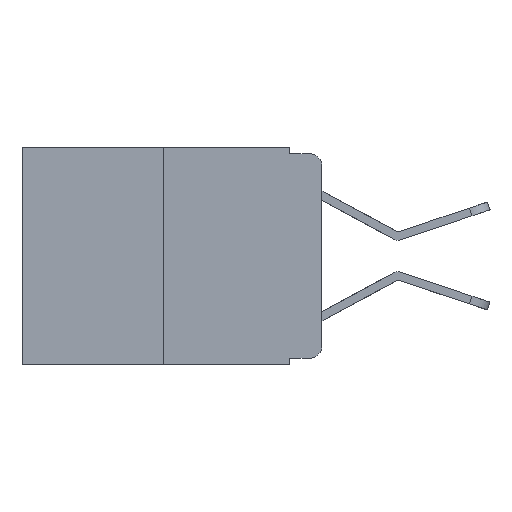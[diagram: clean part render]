
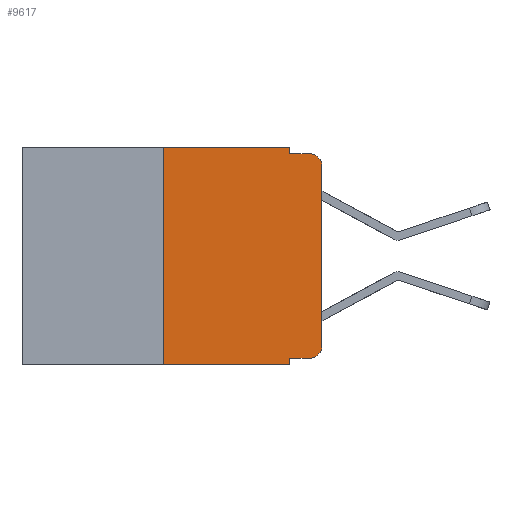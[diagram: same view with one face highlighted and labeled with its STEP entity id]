
A CAD part, left-side view. The second image highlights one B-rep face of the part: STEP entity #9617.
In plain terms, the highlighted planar face has unit normal (-1, 0, 0).
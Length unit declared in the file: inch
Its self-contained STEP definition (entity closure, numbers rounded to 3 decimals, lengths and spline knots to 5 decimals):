
#63 = EDGE_CURVE ( 'NONE', #12526, #5836, #4943, .T. ) ;
#164 = CARTESIAN_POINT ( 'NONE',  ( 0., 0.051, -0.333 ) ) ;
#312 = CIRCLE ( 'NONE', #6295, 0.02 ) ;
#563 = EDGE_CURVE ( 'NONE', #21910, #14165, #8749, .T. ) ;
#1496 = VERTEX_POINT ( 'NONE', #6691 ) ;
#2004 = ORIENTED_EDGE ( 'NONE', *, *, #4461, .T. ) ;
#2182 = VERTEX_POINT ( 'NONE', #14511 ) ;
#2661 = EDGE_CURVE ( 'NONE', #5836, #21910, #312, .T. ) ;
#2753 = DIRECTION ( 'NONE',  ( 1., 0., 0. ) ) ;
#2936 = ORIENTED_EDGE ( 'NONE', *, *, #20538, .F. ) ;
#3021 = CARTESIAN_POINT ( 'NONE',  ( 0., 0.02, -0.01 ) ) ;
#3452 = CARTESIAN_POINT ( 'NONE',  ( 0., 0.473, -0.343 ) ) ;
#3718 = VECTOR ( 'NONE', #7671, 39.37008 ) ;
#3837 = ORIENTED_EDGE ( 'NONE', *, *, #11950, .F. ) ;
#4069 = VECTOR ( 'NONE', #9968, 39.37008 ) ;
#4179 = DIRECTION ( 'NONE',  ( 0., -1., 0. ) ) ;
#4271 = CARTESIAN_POINT ( 'NONE',  ( 0., 0., 0. ) ) ;
#4301 = CARTESIAN_POINT ( 'NONE',  ( 0., 0.051, -0.01 ) ) ;
#4461 = EDGE_CURVE ( 'NONE', #14165, #23490, #7382, .T. ) ;
#4800 = EDGE_CURVE ( 'NONE', #9645, #7943, #13413, .T. ) ;
#4835 = DIRECTION ( 'NONE',  ( 0., 0., -1. ) ) ;
#4943 = LINE ( 'NONE', #164, #14224 ) ;
#5039 = ORIENTED_EDGE ( 'NONE', *, *, #4800, .F. ) ;
#5061 = VECTOR ( 'NONE', #20917, 39.37008 ) ;
#5350 = ORIENTED_EDGE ( 'NONE', *, *, #2661, .T. ) ;
#5836 = VERTEX_POINT ( 'NONE', #7861 ) ;
#6080 = LINE ( 'NONE', #14783, #20193 ) ;
#6223 = EDGE_LOOP ( 'NONE', ( #20037, #2004, #22327, #3837, #5039, #19759, #6235, #2936, #18343, #5350 ) ) ;
#6235 = ORIENTED_EDGE ( 'NONE', *, *, #7889, .T. ) ;
#6295 = AXIS2_PLACEMENT_3D ( 'NONE', #12058, #17781, #4835 ) ;
#6691 = CARTESIAN_POINT ( 'NONE',  ( 0., 0.051, -0.343 ) ) ;
#7240 = LINE ( 'NONE', #3452, #12711 ) ;
#7382 = CIRCLE ( 'NONE', #22490, 0.02 ) ;
#7671 = DIRECTION ( 'NONE',  ( 0., 0., 1. ) ) ;
#7861 = CARTESIAN_POINT ( 'NONE',  ( 0., 0.02, -0.333 ) ) ;
#7889 = EDGE_CURVE ( 'NONE', #2182, #1496, #7240, .T. ) ;
#7943 = VERTEX_POINT ( 'NONE', #23871 ) ;
#8057 = DIRECTION ( 'NONE',  ( -1., 0., 0. ) ) ;
#8116 = DIRECTION ( 'NONE',  ( 0., 0., -1. ) ) ;
#8134 = CARTESIAN_POINT ( 'NONE',  ( 0., 0.02, -0.03 ) ) ;
#8174 = DIRECTION ( 'NONE',  ( 0., 0., -1. ) ) ;
#8749 = LINE ( 'NONE', #4271, #3718 ) ;
#9491 = EDGE_CURVE ( 'NONE', #21548, #23490, #14929, .T. ) ;
#9617 = ADVANCED_FACE ( 'NONE', ( #18067 ), #21228, .F. ) ;
#9645 = VERTEX_POINT ( 'NONE', #21305 ) ;
#9955 = LINE ( 'NONE', #20974, #14245 ) ;
#9968 = DIRECTION ( 'NONE',  ( 0., -1., 0. ) ) ;
#11950 = EDGE_CURVE ( 'NONE', #7943, #21548, #9955, .T. ) ;
#12058 = CARTESIAN_POINT ( 'NONE',  ( 0., 0.02, -0.313 ) ) ;
#12369 = CARTESIAN_POINT ( 'NONE',  ( 0., 0.473, 0. ) ) ;
#12526 = VERTEX_POINT ( 'NONE', #23501 ) ;
#12624 = CARTESIAN_POINT ( 'NONE',  ( 0., 0.051, 0. ) ) ;
#12711 = VECTOR ( 'NONE', #16442, 39.37008 ) ;
#13193 = EDGE_CURVE ( 'NONE', #2182, #9645, #6080, .T. ) ;
#13413 = LINE ( 'NONE', #12369, #4069 ) ;
#13960 = CARTESIAN_POINT ( 'NONE',  ( 0., 0.473, 0. ) ) ;
#14165 = VERTEX_POINT ( 'NONE', #21274 ) ;
#14224 = VECTOR ( 'NONE', #4179, 39.37008 ) ;
#14245 = VECTOR ( 'NONE', #8174, 39.37008 ) ;
#14462 = DIRECTION ( 'NONE',  ( 0., 0., -1. ) ) ;
#14511 = CARTESIAN_POINT ( 'NONE',  ( 0., 0.25, -0.343 ) ) ;
#14610 = LINE ( 'NONE', #12624, #23753 ) ;
#14783 = CARTESIAN_POINT ( 'NONE',  ( 0., 0.25, 0. ) ) ;
#14929 = LINE ( 'NONE', #4301, #5061 ) ;
#15791 = DIRECTION ( 'NONE',  ( 0., 0., -1. ) ) ;
#15836 = CARTESIAN_POINT ( 'NONE',  ( 0., 0.051, -0.01 ) ) ;
#16442 = DIRECTION ( 'NONE',  ( 0., -1., 0. ) ) ;
#16616 = DIRECTION ( 'NONE',  ( 0., 0., 1. ) ) ;
#17781 = DIRECTION ( 'NONE',  ( -1., 0., 0. ) ) ;
#18067 = FACE_OUTER_BOUND ( 'NONE', #6223, .T. ) ;
#18343 = ORIENTED_EDGE ( 'NONE', *, *, #63, .T. ) ;
#19759 = ORIENTED_EDGE ( 'NONE', *, *, #13193, .F. ) ;
#19985 = AXIS2_PLACEMENT_3D ( 'NONE', #13960, #2753, #15791 ) ;
#20037 = ORIENTED_EDGE ( 'NONE', *, *, #563, .T. ) ;
#20193 = VECTOR ( 'NONE', #16616, 39.37008 ) ;
#20538 = EDGE_CURVE ( 'NONE', #12526, #1496, #14610, .T. ) ;
#20917 = DIRECTION ( 'NONE',  ( 0., -1., 0. ) ) ;
#20974 = CARTESIAN_POINT ( 'NONE',  ( 0., 0.051, 0. ) ) ;
#21228 = PLANE ( 'NONE',  #19985 ) ;
#21274 = CARTESIAN_POINT ( 'NONE',  ( 0., 0., -0.03 ) ) ;
#21305 = CARTESIAN_POINT ( 'NONE',  ( 0., 0.25, 0. ) ) ;
#21548 = VERTEX_POINT ( 'NONE', #15836 ) ;
#21910 = VERTEX_POINT ( 'NONE', #22297 ) ;
#22297 = CARTESIAN_POINT ( 'NONE',  ( 0., 0., -0.313 ) ) ;
#22327 = ORIENTED_EDGE ( 'NONE', *, *, #9491, .F. ) ;
#22490 = AXIS2_PLACEMENT_3D ( 'NONE', #8134, #8057, #8116 ) ;
#23490 = VERTEX_POINT ( 'NONE', #3021 ) ;
#23501 = CARTESIAN_POINT ( 'NONE',  ( 0., 0.051, -0.333 ) ) ;
#23753 = VECTOR ( 'NONE', #14462, 39.37008 ) ;
#23871 = CARTESIAN_POINT ( 'NONE',  ( 0., 0.051, 0. ) ) ;
